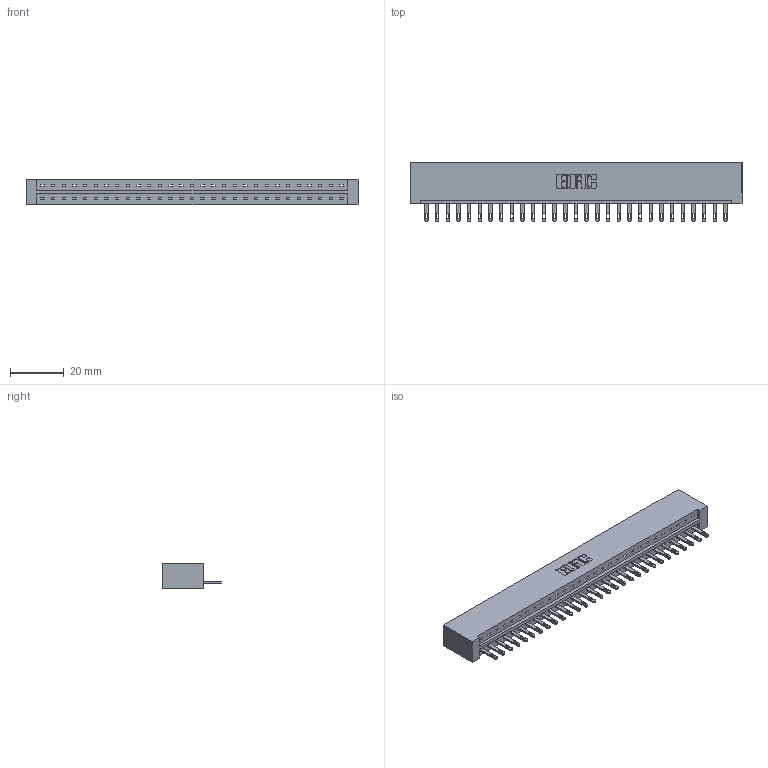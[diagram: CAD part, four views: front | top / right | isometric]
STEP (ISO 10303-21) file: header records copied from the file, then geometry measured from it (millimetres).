
FILE_DESCRIPTION (( 'STEP AP203' ), '1' );
FILE_NAME ('333-029-500-101.STEP', '2018-08-02T16:05:30', ( '' ), ( '' ), 'SwSTEP 2.0', 'SolidWorks 2016', '' );
FILE_SCHEMA (( 'CONFIG_CONTROL_DESIGN' ));
Length unit declared in the file: inch
Products named in the file (3): 333 Part_Lugless; 345-292-001_345-293-100; 333-029-500-101
Assembly tree (30 placements, depth 2):
  333-029-500-101
    333 Part_Lugless
    345-292-001_345-293-100  x29
Bounding box: 123.16 x 21.85 x 9.4 mm (x, y, z)
Volume: 12912.7 mm3; surface area: 13913.2 mm2
Topology: 30 solids, 30 shells, 1672 faces, 5159 edges, 3438 vertices
Faces by surface type: plane 1110, cylinder 562
Entity records: 19063 total; most frequent: CARTESIAN_POINT 3297, ORIENTED_EDGE 3262, DIRECTION 2801, EDGE_CURVE 1631, VECTOR 1507, LINE 1507, VERTEX_POINT 1086, AXIS2_PLACEMENT_3D 647
